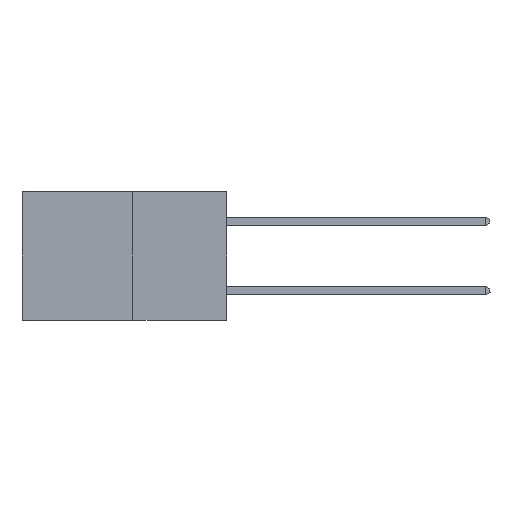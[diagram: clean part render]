
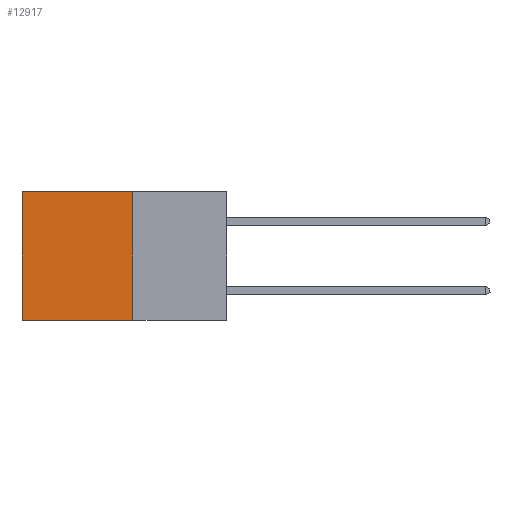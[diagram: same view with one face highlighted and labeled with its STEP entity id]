
A CAD part, left-side view. The second image highlights one B-rep face of the part: STEP entity #12917.
In plain terms, the highlighted planar face has unit normal (-1, 0, 0).
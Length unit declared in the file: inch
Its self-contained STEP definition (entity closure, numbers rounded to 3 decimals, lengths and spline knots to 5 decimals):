
#951 = DIRECTION ( 'NONE',  ( 0., 0., -1. ) ) ;
#1547 = CARTESIAN_POINT ( 'NONE',  ( 0.277, 0.27, 0. ) ) ;
#1706 = CARTESIAN_POINT ( 'NONE',  ( 0.277, 0.27, -0.37 ) ) ;
#1833 = DIRECTION ( 'NONE',  ( 1., 0., 0. ) ) ;
#3297 = PLANE ( 'NONE',  #14810 ) ;
#3484 = LINE ( 'NONE', #5359, #19262 ) ;
#4075 = VECTOR ( 'NONE', #951, 39.37008 ) ;
#4094 = LINE ( 'NONE', #18577, #19375 ) ;
#4595 = ORIENTED_EDGE ( 'NONE', *, *, #12652, .F. ) ;
#4734 = ORIENTED_EDGE ( 'NONE', *, *, #5230, .T. ) ;
#5095 = VERTEX_POINT ( 'NONE', #1547 ) ;
#5230 = EDGE_CURVE ( 'NONE', #11386, #8601, #4094, .T. ) ;
#5359 = CARTESIAN_POINT ( 'NONE',  ( 0.277, 0.27, -0.37 ) ) ;
#6978 = DIRECTION ( 'NONE',  ( 0., 1., 0. ) ) ;
#7116 = ORIENTED_EDGE ( 'NONE', *, *, #17984, .F. ) ;
#8046 = DIRECTION ( 'NONE',  ( 0., 1., 0. ) ) ;
#8601 = VERTEX_POINT ( 'NONE', #8882 ) ;
#8702 = CARTESIAN_POINT ( 'NONE',  ( 0.277, 0.27, -0.37 ) ) ;
#8882 = CARTESIAN_POINT ( 'NONE',  ( 0.277, 0.59, -0.37 ) ) ;
#11085 = CARTESIAN_POINT ( 'NONE',  ( 0.277, 0.27, -0.37 ) ) ;
#11386 = VERTEX_POINT ( 'NONE', #13393 ) ;
#11580 = ORIENTED_EDGE ( 'NONE', *, *, #19081, .T. ) ;
#11986 = LINE ( 'NONE', #17141, #12464 ) ;
#12464 = VECTOR ( 'NONE', #8046, 39.37008 ) ;
#12589 = DIRECTION ( 'NONE',  ( 0., 0., -1. ) ) ;
#12652 = EDGE_CURVE ( 'NONE', #18993, #8601, #3484, .T. ) ;
#12917 = ADVANCED_FACE ( 'NONE', ( #14576 ), #3297, .F. ) ;
#13393 = CARTESIAN_POINT ( 'NONE',  ( 0.277, 0.59, 0. ) ) ;
#13476 = EDGE_LOOP ( 'NONE', ( #4734, #4595, #7116, #11580 ) ) ;
#14576 = FACE_OUTER_BOUND ( 'NONE', #13476, .T. ) ;
#14810 = AXIS2_PLACEMENT_3D ( 'NONE', #11085, #1833, #12589 ) ;
#16311 = LINE ( 'NONE', #8702, #4075 ) ;
#17141 = CARTESIAN_POINT ( 'NONE',  ( 0.277, 0.27, 0. ) ) ;
#17984 = EDGE_CURVE ( 'NONE', #5095, #18993, #16311, .T. ) ;
#18577 = CARTESIAN_POINT ( 'NONE',  ( 0.277, 0.59, -0.37 ) ) ;
#18993 = VERTEX_POINT ( 'NONE', #1706 ) ;
#19081 = EDGE_CURVE ( 'NONE', #5095, #11386, #11986, .T. ) ;
#19262 = VECTOR ( 'NONE', #6978, 39.37008 ) ;
#19375 = VECTOR ( 'NONE', #19632, 39.37008 ) ;
#19632 = DIRECTION ( 'NONE',  ( 0., 0., -1. ) ) ;
